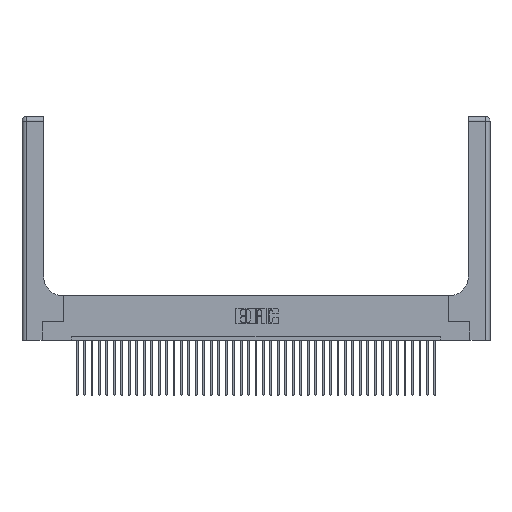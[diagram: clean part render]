
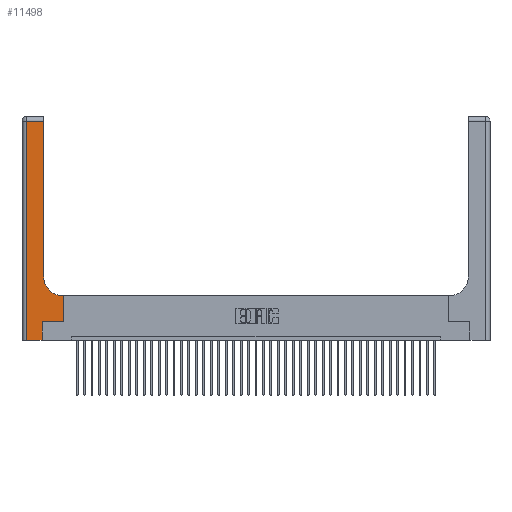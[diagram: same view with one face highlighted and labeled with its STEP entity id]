
A CAD part, top view. The second image highlights one B-rep face of the part: STEP entity #11498.
In plain terms, the highlighted planar face has unit normal (0, 0, 1).
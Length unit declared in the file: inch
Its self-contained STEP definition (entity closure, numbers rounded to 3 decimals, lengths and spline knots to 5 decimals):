
#216 = CARTESIAN_POINT ( 'NONE',  ( 0., 0., 0.37 ) ) ;
#329 = ORIENTED_EDGE ( 'NONE', *, *, #30800, .T. ) ;
#608 = LINE ( 'NONE', #38484, #14565 ) ;
#780 = VECTOR ( 'NONE', #8101, 39.37008 ) ;
#1243 = EDGE_CURVE ( 'NONE', #14953, #12266, #38175, .T. ) ;
#2200 = DIRECTION ( 'NONE',  ( 0., 1., 0. ) ) ;
#2290 = ORIENTED_EDGE ( 'NONE', *, *, #34348, .T. ) ;
#2647 = CARTESIAN_POINT ( 'NONE',  ( 0.5585, 0.25, 0.37 ) ) ;
#3873 = DIRECTION ( 'NONE',  ( 0., -1., 0. ) ) ;
#4862 = ORIENTED_EDGE ( 'NONE', *, *, #30025, .T. ) ;
#6747 = ORIENTED_EDGE ( 'NONE', *, *, #10219, .T. ) ;
#7667 = LINE ( 'NONE', #9386, #10605 ) ;
#7778 = CARTESIAN_POINT ( 'NONE',  ( 0.5585, 0.6, 0.37 ) ) ;
#8101 = DIRECTION ( 'NONE',  ( 0., 1., 0. ) ) ;
#8193 = VERTEX_POINT ( 'NONE', #19929 ) ;
#8228 = ORIENTED_EDGE ( 'NONE', *, *, #1243, .T. ) ;
#8267 = DIRECTION ( 'NONE',  ( -1., 0., 0. ) ) ;
#8627 = CARTESIAN_POINT ( 'NONE',  ( 0.2915, 2.94, 0.37 ) ) ;
#9386 = CARTESIAN_POINT ( 'NONE',  ( 0.06, 3., 0.37 ) ) ;
#9437 = DIRECTION ( 'NONE',  ( -1., 0., 0. ) ) ;
#9945 = LINE ( 'NONE', #23361, #11505 ) ;
#10200 = EDGE_LOOP ( 'NONE', ( #2290, #329, #16325, #8228, #22840, #4862, #6747, #11183, #34763 ) ) ;
#10219 = EDGE_CURVE ( 'NONE', #35703, #20226, #16629, .T. ) ;
#10605 = VECTOR ( 'NONE', #3873, 39.37008 ) ;
#10724 = DIRECTION ( 'NONE',  ( -1., 0., 0. ) ) ;
#10840 = VERTEX_POINT ( 'NONE', #8627 ) ;
#11068 = DIRECTION ( 'NONE',  ( 0., 1., 0. ) ) ;
#11183 = ORIENTED_EDGE ( 'NONE', *, *, #30956, .T. ) ;
#11199 = PLANE ( 'NONE',  #24305 ) ;
#11469 = CARTESIAN_POINT ( 'NONE',  ( 0.5585, 0.25, 0.37 ) ) ;
#11498 = ADVANCED_FACE ( 'NONE', ( #37535 ), #11199, .F. ) ;
#11505 = VECTOR ( 'NONE', #10724, 39.37008 ) ;
#12068 = CARTESIAN_POINT ( 'NONE',  ( 0.06, 0., 0.37 ) ) ;
#12116 = CARTESIAN_POINT ( 'NONE',  ( 0.5415, 0.85, 0.37 ) ) ;
#12266 = VERTEX_POINT ( 'NONE', #33187 ) ;
#12897 = VECTOR ( 'NONE', #8267, 39.37008 ) ;
#13175 = EDGE_CURVE ( 'NONE', #18394, #8193, #28783, .T. ) ;
#13711 = VERTEX_POINT ( 'NONE', #40516 ) ;
#14484 = LINE ( 'NONE', #18003, #12897 ) ;
#14565 = VECTOR ( 'NONE', #31498, 39.37008 ) ;
#14953 = VERTEX_POINT ( 'NONE', #12068 ) ;
#15057 = EDGE_CURVE ( 'NONE', #12266, #13711, #35291, .T. ) ;
#15962 = DIRECTION ( 'NONE',  ( 0., 0., -1. ) ) ;
#16325 = ORIENTED_EDGE ( 'NONE', *, *, #17914, .T. ) ;
#16629 = LINE ( 'NONE', #11469, #21641 ) ;
#17914 = EDGE_CURVE ( 'NONE', #30556, #14953, #7667, .T. ) ;
#18003 = CARTESIAN_POINT ( 'NONE',  ( 0.2915, 0.6, 0.37 ) ) ;
#18394 = VERTEX_POINT ( 'NONE', #33743 ) ;
#19929 = CARTESIAN_POINT ( 'NONE',  ( 0.2915, 0.85, 0.37 ) ) ;
#20226 = VERTEX_POINT ( 'NONE', #7778 ) ;
#20411 = CARTESIAN_POINT ( 'NONE',  ( 0.269, 0., 0.37 ) ) ;
#21641 = VECTOR ( 'NONE', #2200, 39.37008 ) ;
#22840 = ORIENTED_EDGE ( 'NONE', *, *, #15057, .T. ) ;
#23361 = CARTESIAN_POINT ( 'NONE',  ( 0., 2.94, 0.37 ) ) ;
#24305 = AXIS2_PLACEMENT_3D ( 'NONE', #33467, #26538, #9437 ) ;
#24532 = CARTESIAN_POINT ( 'NONE',  ( 0.06, 2.94, 0.37 ) ) ;
#26538 = DIRECTION ( 'NONE',  ( 0., 0., -1. ) ) ;
#26829 = DIRECTION ( 'NONE',  ( 1., 0., 0. ) ) ;
#27432 = CARTESIAN_POINT ( 'NONE',  ( 0.2915, 3., 0.37 ) ) ;
#28783 = CIRCLE ( 'NONE', #38667, 0.25 ) ;
#30025 = EDGE_CURVE ( 'NONE', #13711, #35703, #608, .T. ) ;
#30556 = VERTEX_POINT ( 'NONE', #24532 ) ;
#30692 = LINE ( 'NONE', #27432, #780 ) ;
#30800 = EDGE_CURVE ( 'NONE', #10840, #30556, #9945, .T. ) ;
#30956 = EDGE_CURVE ( 'NONE', #20226, #18394, #14484, .T. ) ;
#31498 = DIRECTION ( 'NONE',  ( 1., 0., 0. ) ) ;
#33187 = CARTESIAN_POINT ( 'NONE',  ( 0.269, 0., 0.37 ) ) ;
#33467 = CARTESIAN_POINT ( 'NONE',  ( 0., 3., 0.37 ) ) ;
#33743 = CARTESIAN_POINT ( 'NONE',  ( 0.5415, 0.6, 0.37 ) ) ;
#34348 = EDGE_CURVE ( 'NONE', #8193, #10840, #30692, .T. ) ;
#34763 = ORIENTED_EDGE ( 'NONE', *, *, #13175, .T. ) ;
#34856 = VECTOR ( 'NONE', #11068, 39.37008 ) ;
#35291 = LINE ( 'NONE', #20411, #34856 ) ;
#35703 = VERTEX_POINT ( 'NONE', #2647 ) ;
#36212 = VECTOR ( 'NONE', #38405, 39.37008 ) ;
#37535 = FACE_OUTER_BOUND ( 'NONE', #10200, .T. ) ;
#38175 = LINE ( 'NONE', #216, #36212 ) ;
#38405 = DIRECTION ( 'NONE',  ( 1., 0., 0. ) ) ;
#38484 = CARTESIAN_POINT ( 'NONE',  ( 0.269, 0.25, 0.37 ) ) ;
#38667 = AXIS2_PLACEMENT_3D ( 'NONE', #12116, #15962, #26829 ) ;
#40516 = CARTESIAN_POINT ( 'NONE',  ( 0.269, 0.25, 0.37 ) ) ;
